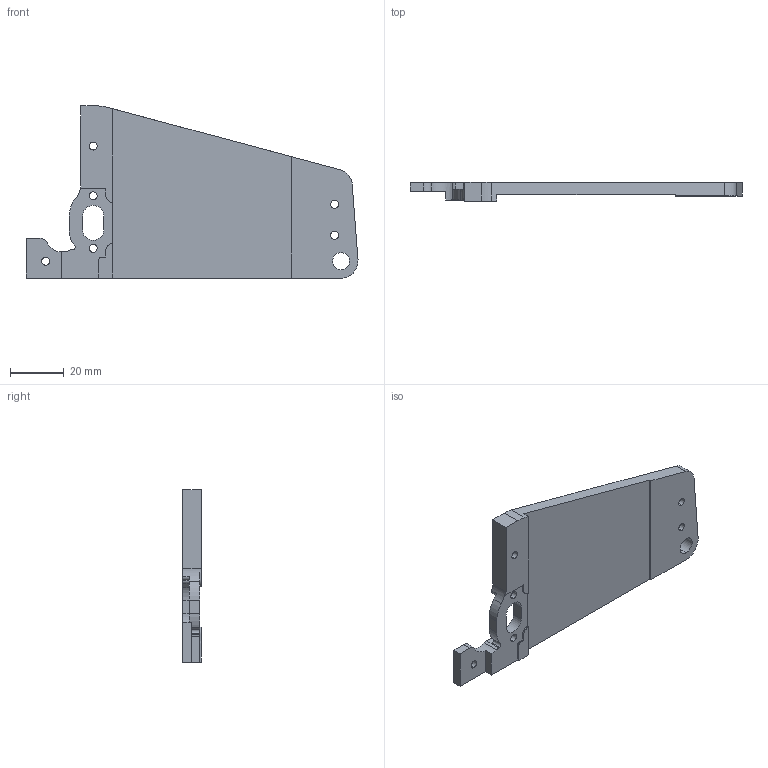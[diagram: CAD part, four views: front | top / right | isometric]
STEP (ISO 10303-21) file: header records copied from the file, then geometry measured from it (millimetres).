
FILE_DESCRIPTION (( 'STEP AP214' ), '1' );
FILE_NAME ('Thunderbolt_Mag_Well_Right_Blank.STEP', '2021-09-12T03:35:34', ( '' ), ( '' ), 'SwSTEP 2.0', 'SolidWorks 2020', '' );
FILE_SCHEMA (( 'AUTOMOTIVE_DESIGN' ));
Length unit declared in the file: millimetre
Products named in the file (1): Thunderbolt_Mag_Well_Right_Blank
Bounding box: 124.11 x 7.03 x 64.36 mm (x, y, z)
Volume: 26003.8 mm3; surface area: 13800.6 mm2
Topology: 1 solids, 1 shells, 105 faces, 297 edges, 198 vertices
Faces by surface type: plane 59, cylinder 46
Entity records: 3493 total; most frequent: DIRECTION 605, CARTESIAN_POINT 601, ORIENTED_EDGE 594, EDGE_CURVE 297, AXIS2_PLACEMENT_3D 202, VECTOR 201, LINE 201, VERTEX_POINT 198
